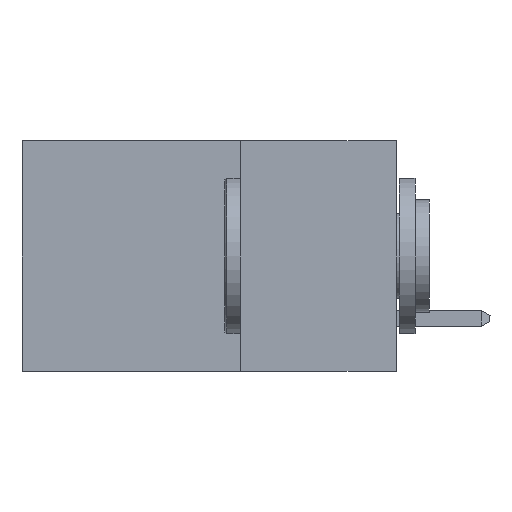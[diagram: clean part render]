
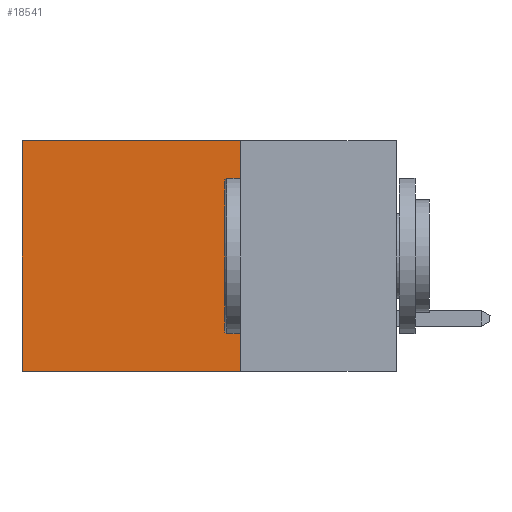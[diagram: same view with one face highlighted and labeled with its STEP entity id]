
A CAD part, left-side view. The second image highlights one B-rep face of the part: STEP entity #18541.
In plain terms, the highlighted planar face has unit normal (-1, 0, 0).
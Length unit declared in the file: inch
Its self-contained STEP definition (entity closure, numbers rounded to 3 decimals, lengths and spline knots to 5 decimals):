
#548 = PLANE ( 'NONE',  #18906 ) ;
#571 = DIRECTION ( 'NONE',  ( 0., 0., -1. ) ) ;
#1307 = VECTOR ( 'NONE', #12938, 39.37008 ) ;
#1432 = LINE ( 'NONE', #12253, #10612 ) ;
#1836 = FACE_OUTER_BOUND ( 'NONE', #20122, .T. ) ;
#2013 = CARTESIAN_POINT ( 'NONE',  ( 0.2615, 0.6, -0.37 ) ) ;
#3583 = DIRECTION ( 'NONE',  ( 0., 1., 0. ) ) ;
#3618 = VECTOR ( 'NONE', #11861, 39.37008 ) ;
#3738 = EDGE_CURVE ( 'NONE', #11426, #20919, #8804, .T. ) ;
#4539 = CARTESIAN_POINT ( 'NONE',  ( 0.2615, 0.25, -0.37 ) ) ;
#6277 = VECTOR ( 'NONE', #3583, 39.37008 ) ;
#6531 = DIRECTION ( 'NONE',  ( 0., 0., -1. ) ) ;
#6589 = LINE ( 'NONE', #9070, #1307 ) ;
#7153 = VERTEX_POINT ( 'NONE', #18934 ) ;
#7198 = EDGE_CURVE ( 'NONE', #7153, #16536, #11377, .T. ) ;
#7702 = CARTESIAN_POINT ( 'NONE',  ( 0.2615, 0.25, 0. ) ) ;
#8804 = LINE ( 'NONE', #11842, #3618 ) ;
#9070 = CARTESIAN_POINT ( 'NONE',  ( 0.2615, 0.25, -0.37 ) ) ;
#10612 = VECTOR ( 'NONE', #571, 39.37008 ) ;
#11377 = LINE ( 'NONE', #22733, #6277 ) ;
#11426 = VERTEX_POINT ( 'NONE', #7702 ) ;
#11842 = CARTESIAN_POINT ( 'NONE',  ( 0.2615, 0.25, 0. ) ) ;
#11861 = DIRECTION ( 'NONE',  ( 0., 1., 0. ) ) ;
#12253 = CARTESIAN_POINT ( 'NONE',  ( 0.2615, 0.6, -0.37 ) ) ;
#12938 = DIRECTION ( 'NONE',  ( 0., 0., -1. ) ) ;
#13384 = ORIENTED_EDGE ( 'NONE', *, *, #23386, .F. ) ;
#14423 = EDGE_CURVE ( 'NONE', #20919, #16536, #1432, .T. ) ;
#16235 = ORIENTED_EDGE ( 'NONE', *, *, #7198, .F. ) ;
#16536 = VERTEX_POINT ( 'NONE', #2013 ) ;
#17066 = CARTESIAN_POINT ( 'NONE',  ( 0.2615, 0.6, 0. ) ) ;
#18096 = DIRECTION ( 'NONE',  ( 1., 0., 0. ) ) ;
#18541 = ADVANCED_FACE ( 'NONE', ( #1836 ), #548, .F. ) ;
#18906 = AXIS2_PLACEMENT_3D ( 'NONE', #4539, #18096, #6531 ) ;
#18934 = CARTESIAN_POINT ( 'NONE',  ( 0.2615, 0.25, -0.37 ) ) ;
#20122 = EDGE_LOOP ( 'NONE', ( #21830, #16235, #13384, #22134 ) ) ;
#20919 = VERTEX_POINT ( 'NONE', #17066 ) ;
#21830 = ORIENTED_EDGE ( 'NONE', *, *, #14423, .T. ) ;
#22134 = ORIENTED_EDGE ( 'NONE', *, *, #3738, .T. ) ;
#22733 = CARTESIAN_POINT ( 'NONE',  ( 0.2615, 0.25, -0.37 ) ) ;
#23386 = EDGE_CURVE ( 'NONE', #11426, #7153, #6589, .T. ) ;
